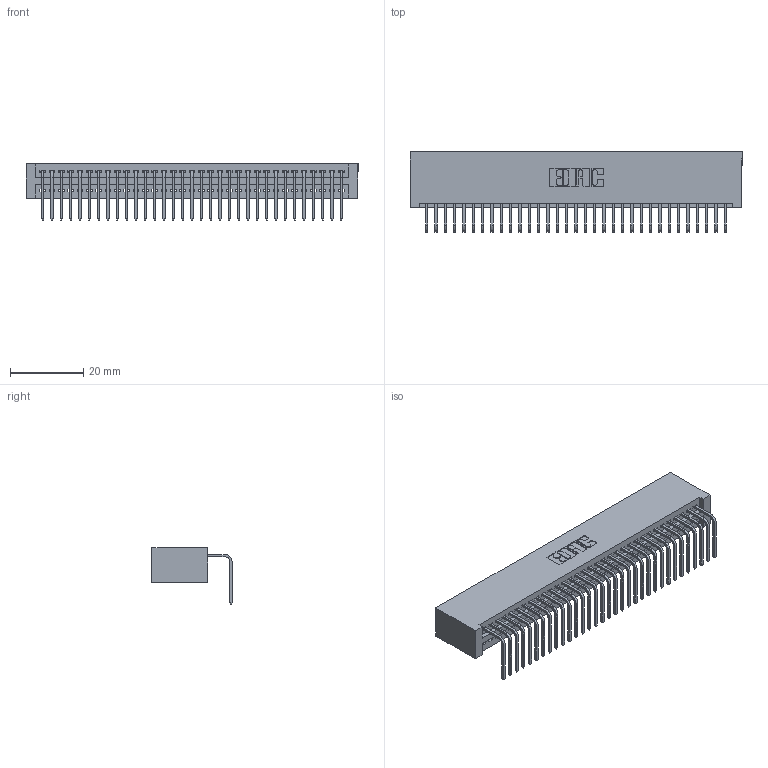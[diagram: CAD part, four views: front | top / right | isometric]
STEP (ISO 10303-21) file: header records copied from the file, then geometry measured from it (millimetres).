
FILE_DESCRIPTION (( 'STEP AP203' ), '1' );
FILE_NAME ('345-033-558-101.STEP', '2018-08-24T12:13:46', ( '' ), ( '' ), 'SwSTEP 2.0', 'SolidWorks 2016', '' );
FILE_SCHEMA (( 'CONFIG_CONTROL_DESIGN' ));
Length unit declared in the file: inch
Products named in the file (3): 345 Part_No Mounting Lugs; 345-292-001_558 Tail - 2; 345-033-558-101
Assembly tree (34 placements, depth 2):
  345-033-558-101
    345 Part_No Mounting Lugs
    345-292-001_558 Tail - 2  x33
Bounding box: 90.42 x 21.83 x 15.37 mm (x, y, z)
Volume: 9209.1 mm3; surface area: 12952 mm2
Topology: 34 solids, 34 shells, 2098 faces, 6323 edges, 4170 vertices
Faces by surface type: plane 1462, cylinder 636
Entity records: 25855 total; most frequent: CARTESIAN_POINT 4487, ORIENTED_EDGE 4454, DIRECTION 3925, EDGE_CURVE 2227, VECTOR 1971, LINE 1971, VERTEX_POINT 1482, AXIS2_PLACEMENT_3D 977
